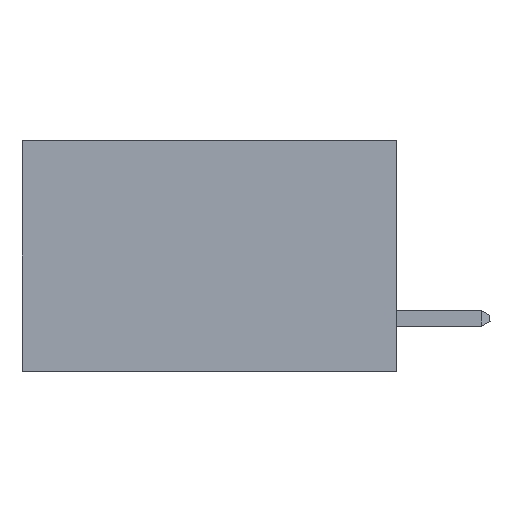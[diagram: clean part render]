
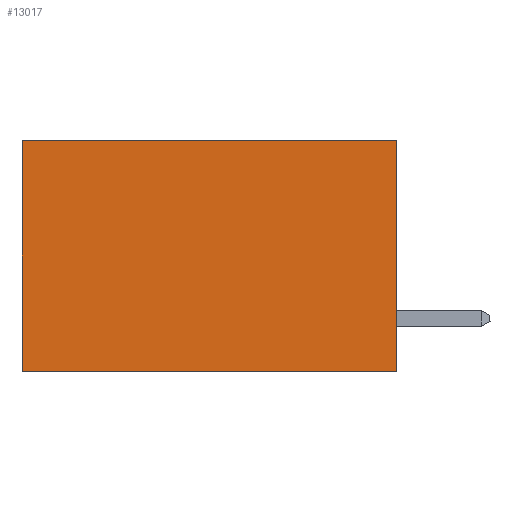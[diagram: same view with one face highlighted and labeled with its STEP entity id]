
A CAD part, left-side view. The second image highlights one B-rep face of the part: STEP entity #13017.
In plain terms, the highlighted planar face has unit normal (-1, 0, 0).
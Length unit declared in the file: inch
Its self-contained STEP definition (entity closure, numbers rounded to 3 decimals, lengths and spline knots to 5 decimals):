
#906 = PLANE ( 'NONE',  #8932 ) ;
#937 = VERTEX_POINT ( 'NONE', #7231 ) ;
#1442 = VECTOR ( 'NONE', #12724, 39.37008 ) ;
#1491 = DIRECTION ( 'NONE',  ( 0., 0., -1. ) ) ;
#1508 = VERTEX_POINT ( 'NONE', #13856 ) ;
#2617 = VECTOR ( 'NONE', #1491, 39.37008 ) ;
#2986 = FACE_OUTER_BOUND ( 'NONE', #6418, .T. ) ;
#3195 = LINE ( 'NONE', #10413, #2617 ) ;
#3296 = CARTESIAN_POINT ( 'NONE',  ( 0.298, 0., 0. ) ) ;
#3297 = VERTEX_POINT ( 'NONE', #3864 ) ;
#3449 = ORIENTED_EDGE ( 'NONE', *, *, #12592, .T. ) ;
#3599 = LINE ( 'NONE', #10242, #1442 ) ;
#3864 = CARTESIAN_POINT ( 'NONE',  ( 0.298, 0., 0. ) ) ;
#5946 = LINE ( 'NONE', #14889, #15147 ) ;
#6418 = EDGE_LOOP ( 'NONE', ( #11719, #8001, #14395, #3449 ) ) ;
#7231 = CARTESIAN_POINT ( 'NONE',  ( 0.298, 0.6, -0.37 ) ) ;
#7613 = EDGE_CURVE ( 'NONE', #1508, #937, #13211, .T. ) ;
#8001 = ORIENTED_EDGE ( 'NONE', *, *, #14534, .F. ) ;
#8932 = AXIS2_PLACEMENT_3D ( 'NONE', #3296, #13479, #16028 ) ;
#10242 = CARTESIAN_POINT ( 'NONE',  ( 0.298, 0., 0. ) ) ;
#10413 = CARTESIAN_POINT ( 'NONE',  ( 0.298, 0., 0. ) ) ;
#10482 = VERTEX_POINT ( 'NONE', #15042 ) ;
#11719 = ORIENTED_EDGE ( 'NONE', *, *, #7613, .T. ) ;
#12144 = CARTESIAN_POINT ( 'NONE',  ( 0.298, 0.6, 0. ) ) ;
#12592 = EDGE_CURVE ( 'NONE', #3297, #1508, #3599, .T. ) ;
#12724 = DIRECTION ( 'NONE',  ( 0., 1., 0. ) ) ;
#12763 = EDGE_CURVE ( 'NONE', #3297, #10482, #3195, .T. ) ;
#13017 = ADVANCED_FACE ( 'NONE', ( #2986 ), #906, .F. ) ;
#13211 = LINE ( 'NONE', #12144, #14606 ) ;
#13434 = DIRECTION ( 'NONE',  ( 0., 0., -1. ) ) ;
#13479 = DIRECTION ( 'NONE',  ( 1., 0., 0. ) ) ;
#13686 = DIRECTION ( 'NONE',  ( 0., 1., 0. ) ) ;
#13856 = CARTESIAN_POINT ( 'NONE',  ( 0.298, 0.6, 0. ) ) ;
#14395 = ORIENTED_EDGE ( 'NONE', *, *, #12763, .F. ) ;
#14534 = EDGE_CURVE ( 'NONE', #10482, #937, #5946, .T. ) ;
#14606 = VECTOR ( 'NONE', #13434, 39.37008 ) ;
#14889 = CARTESIAN_POINT ( 'NONE',  ( 0.298, 0., -0.37 ) ) ;
#15042 = CARTESIAN_POINT ( 'NONE',  ( 0.298, 0., -0.37 ) ) ;
#15147 = VECTOR ( 'NONE', #13686, 39.37008 ) ;
#16028 = DIRECTION ( 'NONE',  ( 0., 0., -1. ) ) ;
